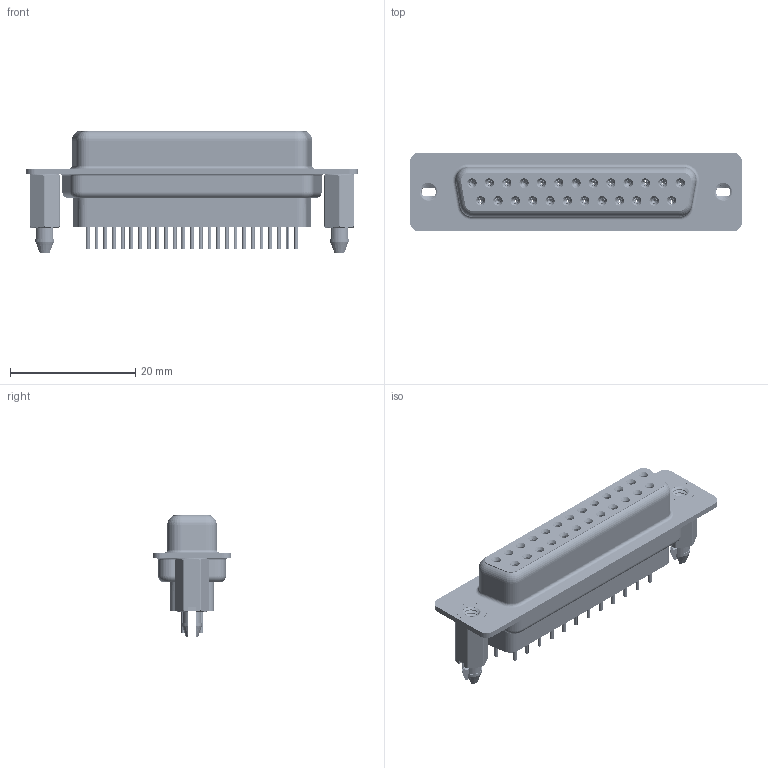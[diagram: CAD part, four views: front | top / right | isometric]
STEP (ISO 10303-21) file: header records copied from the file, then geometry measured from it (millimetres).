
FILE_DESCRIPTION (( 'STEP AP203' ), '1' );
FILE_NAME ('628-025-228-266.STEP', '2020-07-21T13:38:04', ( '' ), ( '' ), 'SwSTEP 2.0', 'SolidWorks 2020', '' );
FILE_SCHEMA (( 'CONFIG_CONTROL_DESIGN' ));
Length unit declared in the file: millimetre
Products named in the file (7): 628-025-228-266; 628 Contact Row 1_28L; 628 Contact Row 2_28L; 628 Housing_25 FF; 628 4-40 Threaded Boardlock_FF; 628 Shell Front_25 Contacts; 628 Shell Rear_25 Contacts
Assembly tree (30 placements, depth 2):
  628-025-228-266
    628 Housing_25 FF
    628 Shell Front_25 Contacts
    628 Shell Rear_25 Contacts
    628 Contact Row 1_28L  x13
    628 Contact Row 2_28L  x12
    628 4-40 Threaded Boardlock_FF  x2
Bounding box: 53 x 12.6 x 19.4 mm (x, y, z)
Volume: 4603.8 mm3; surface area: 10933.2 mm2
Topology: 31 solids, 31 shells, 3671 faces, 9438 edges, 5888 vertices
Faces by surface type: cylinder 1083, plane 880, torus 713, bspline 554, cone 441
Entity records: 46795 total; most frequent: CARTESIAN_POINT 23168, DIRECTION 4765, ORIENTED_EDGE 4602, EDGE_CURVE 2301, AXIS2_PLACEMENT_3D 1972, VERTEX_POINT 1464, EDGE_LOOP 1131, CIRCLE 1072
